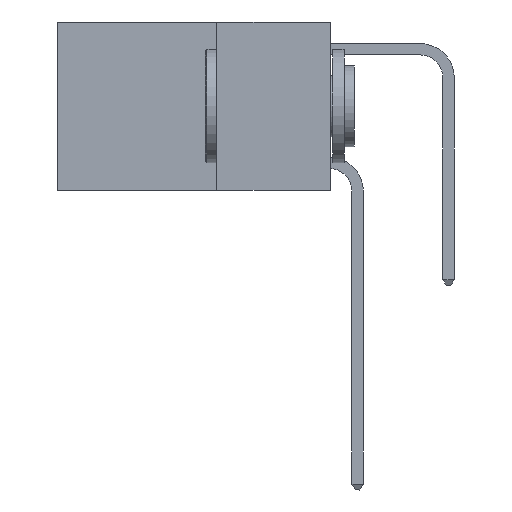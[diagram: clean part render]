
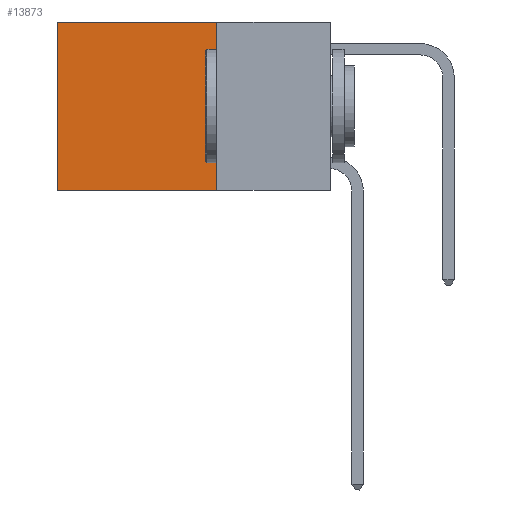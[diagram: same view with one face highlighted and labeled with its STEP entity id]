
A CAD part, left-side view. The second image highlights one B-rep face of the part: STEP entity #13873.
In plain terms, the highlighted planar face has unit normal (-1, 0, 0).
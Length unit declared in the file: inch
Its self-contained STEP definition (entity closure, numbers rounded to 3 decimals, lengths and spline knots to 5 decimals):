
#93 = CARTESIAN_POINT ( 'NONE',  ( 0.2625, 0.25, -0.37 ) ) ;
#292 = EDGE_CURVE ( 'NONE', #8029, #11407, #9359, .T. ) ;
#855 = LINE ( 'NONE', #6431, #5974 ) ;
#1429 = FACE_OUTER_BOUND ( 'NONE', #10911, .T. ) ;
#1570 = DIRECTION ( 'NONE',  ( 1., 0., 0. ) ) ;
#1636 = CARTESIAN_POINT ( 'NONE',  ( 0.2625, 0.6, 0. ) ) ;
#2125 = CARTESIAN_POINT ( 'NONE',  ( 0.2625, 0.25, -0.37 ) ) ;
#2490 = EDGE_CURVE ( 'NONE', #3788, #2734, #855, .T. ) ;
#2734 = VERTEX_POINT ( 'NONE', #2125 ) ;
#3207 = CARTESIAN_POINT ( 'NONE',  ( 0.2625, 0.25, 0. ) ) ;
#3309 = VECTOR ( 'NONE', #6256, 39.37008 ) ;
#3788 = VERTEX_POINT ( 'NONE', #3207 ) ;
#4804 = CARTESIAN_POINT ( 'NONE',  ( 0.2625, 0.25, 0. ) ) ;
#4973 = ORIENTED_EDGE ( 'NONE', *, *, #2490, .F. ) ;
#5208 = ORIENTED_EDGE ( 'NONE', *, *, #7221, .F. ) ;
#5974 = VECTOR ( 'NONE', #9741, 39.37008 ) ;
#6068 = ORIENTED_EDGE ( 'NONE', *, *, #292, .T. ) ;
#6256 = DIRECTION ( 'NONE',  ( 0., 1., 0. ) ) ;
#6431 = CARTESIAN_POINT ( 'NONE',  ( 0.2625, 0.25, 0. ) ) ;
#7221 = EDGE_CURVE ( 'NONE', #2734, #11407, #7781, .T. ) ;
#7322 = VECTOR ( 'NONE', #13305, 39.37008 ) ;
#7781 = LINE ( 'NONE', #93, #7322 ) ;
#7846 = CARTESIAN_POINT ( 'NONE',  ( 0.2625, 0.6, -0.37 ) ) ;
#8029 = VERTEX_POINT ( 'NONE', #11314 ) ;
#8290 = DIRECTION ( 'NONE',  ( 0., 0., -1. ) ) ;
#8829 = ORIENTED_EDGE ( 'NONE', *, *, #9022, .T. ) ;
#9022 = EDGE_CURVE ( 'NONE', #3788, #8029, #11707, .T. ) ;
#9359 = LINE ( 'NONE', #1636, #11035 ) ;
#9741 = DIRECTION ( 'NONE',  ( 0., 0., -1. ) ) ;
#10230 = PLANE ( 'NONE',  #10601 ) ;
#10601 = AXIS2_PLACEMENT_3D ( 'NONE', #4804, #1570, #13160 ) ;
#10692 = CARTESIAN_POINT ( 'NONE',  ( 0.2625, 0.25, 0. ) ) ;
#10911 = EDGE_LOOP ( 'NONE', ( #6068, #5208, #4973, #8829 ) ) ;
#11035 = VECTOR ( 'NONE', #8290, 39.37008 ) ;
#11314 = CARTESIAN_POINT ( 'NONE',  ( 0.2625, 0.6, 0. ) ) ;
#11407 = VERTEX_POINT ( 'NONE', #7846 ) ;
#11707 = LINE ( 'NONE', #10692, #3309 ) ;
#13160 = DIRECTION ( 'NONE',  ( 0., 0., -1. ) ) ;
#13305 = DIRECTION ( 'NONE',  ( 0., 1., 0. ) ) ;
#13873 = ADVANCED_FACE ( 'NONE', ( #1429 ), #10230, .F. ) ;
